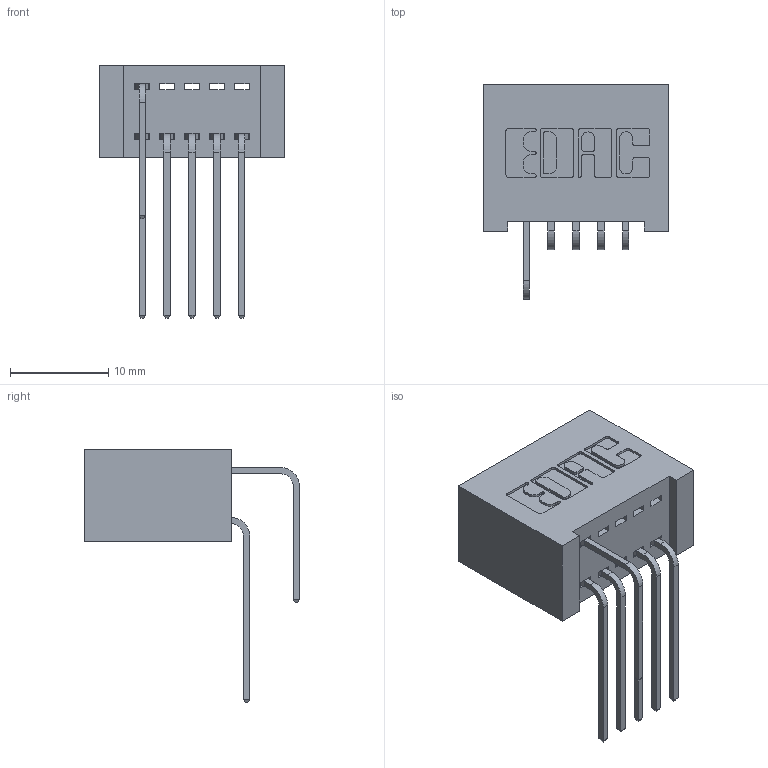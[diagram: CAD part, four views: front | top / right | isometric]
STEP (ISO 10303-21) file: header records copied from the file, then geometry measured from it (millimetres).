
FILE_DESCRIPTION (( 'STEP AP203' ), '1' );
FILE_NAME ('342-010-558-201.STEP', '2018-08-10T14:01:24', ( '' ), ( '' ), 'SwSTEP 2.0', 'SolidWorks 2016', '' );
FILE_SCHEMA (( 'CONFIG_CONTROL_DESIGN' ));
Length unit declared in the file: inch
Products named in the file (4): 342 Part_Lugless; 345-292-001_558 559 Tail - 1; 345-292-001_558 Tail - 2; 342-010-558-201
Assembly tree (7 placements, depth 2):
  342-010-558-201
    342 Part_Lugless
    345-292-001_558 559 Tail - 1  x5
    345-292-001_558 Tail - 2
Bounding box: 18.95 x 21.91 x 25.78 mm (x, y, z)
Volume: 1965.5 mm3; surface area: 2691.5 mm2
Topology: 7 solids, 7 shells, 450 faces, 1325 edges, 874 vertices
Faces by surface type: plane 314, cylinder 136
Entity records: 9249 total; most frequent: CARTESIAN_POINT 1641, ORIENTED_EDGE 1530, DIRECTION 1437, EDGE_CURVE 765, VECTOR 605, LINE 605, VERTEX_POINT 506, AXIS2_PLACEMENT_3D 416
